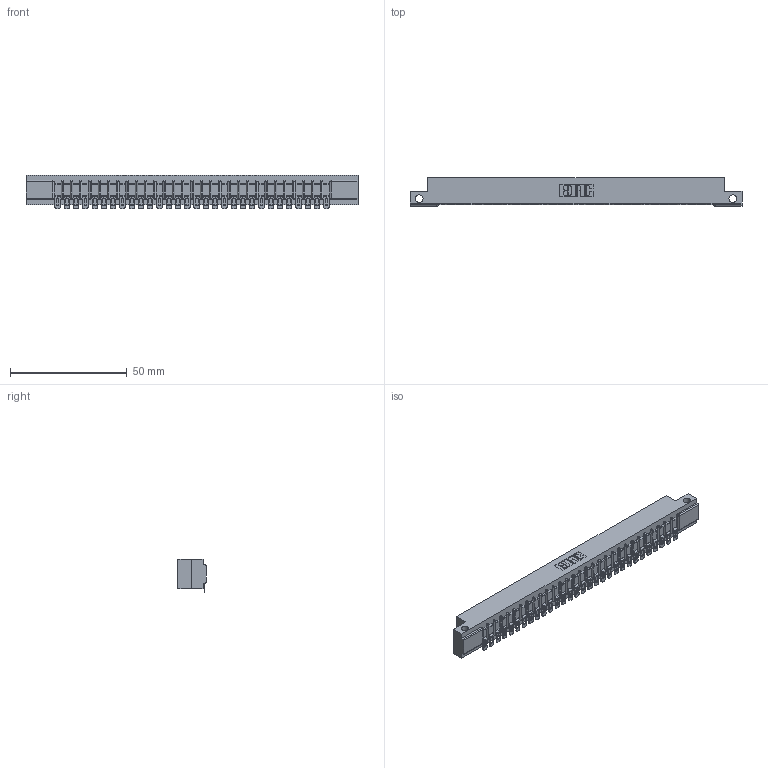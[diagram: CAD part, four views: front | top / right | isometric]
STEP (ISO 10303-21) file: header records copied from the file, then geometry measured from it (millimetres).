
FILE_DESCRIPTION (( 'STEP AP203' ), '1' );
FILE_NAME ('357-030-554-112.STEP', '2019-09-17T03:22:59', ( '' ), ( '' ), 'SwSTEP 2.0', 'SolidWorks 2016', '' );
FILE_SCHEMA (( 'CONFIG_CONTROL_DESIGN' ));
Length unit declared in the file: inch
Products named in the file (3): 307-290-002_554; 357-030-554-112; 307 Part_.128 Dia Side Mounting Holes
Assembly tree (31 placements, depth 2):
  357-030-554-112
    307 Part_.128 Dia Side Mounting Holes
    307-290-002_554  x30
Bounding box: 141.88 x 12.01 x 14.52 mm (x, y, z)
Volume: 14962.6 mm3; surface area: 18655.4 mm2
Topology: 31 solids, 31 shells, 2579 faces, 7913 edges, 5190 vertices
Faces by surface type: plane 1450, cylinder 1067, sphere 62
Entity records: 28165 total; most frequent: CARTESIAN_POINT 4750, ORIENTED_EDGE 4740, DIRECTION 4626, EDGE_CURVE 2370, LINE 1802, VECTOR 1802, VERTEX_POINT 1536, AXIS2_PLACEMENT_3D 1412
